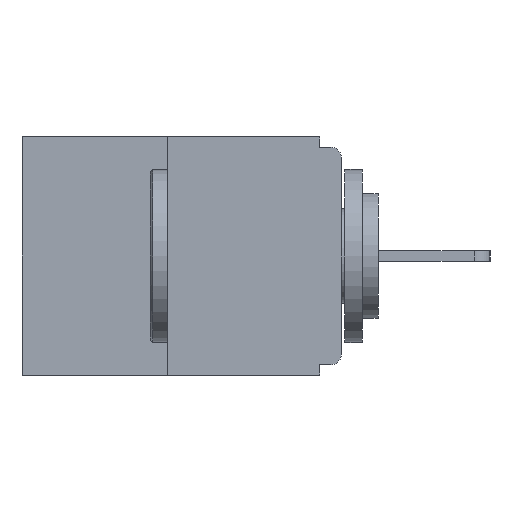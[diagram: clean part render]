
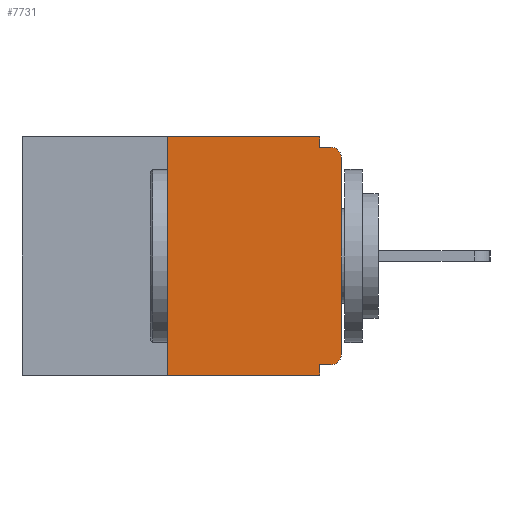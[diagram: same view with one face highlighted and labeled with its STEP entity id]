
A CAD part, left-side view. The second image highlights one B-rep face of the part: STEP entity #7731.
In plain terms, the highlighted planar face has unit normal (-1, 0, 0).
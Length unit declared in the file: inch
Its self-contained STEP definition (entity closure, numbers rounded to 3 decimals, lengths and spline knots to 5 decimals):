
#279 = VECTOR ( 'NONE', #20428, 39.37008 ) ;
#307 = CARTESIAN_POINT ( 'NONE',  ( 0., 0.015, -0.03 ) ) ;
#452 = DIRECTION ( 'NONE',  ( 0., -1., 0. ) ) ;
#669 = ORIENTED_EDGE ( 'NONE', *, *, #16260, .T. ) ;
#897 = VECTOR ( 'NONE', #19097, 39.37008 ) ;
#960 = EDGE_CURVE ( 'NONE', #13443, #11929, #16025, .T. ) ;
#2563 = DIRECTION ( 'NONE',  ( 0., 0., -1. ) ) ;
#2791 = CARTESIAN_POINT ( 'NONE',  ( 0., 0.46, 0. ) ) ;
#3746 = VERTEX_POINT ( 'NONE', #24439 ) ;
#3871 = VECTOR ( 'NONE', #7969, 39.37008 ) ;
#4039 = CARTESIAN_POINT ( 'NONE',  ( 0., 0., -0.328 ) ) ;
#4362 = EDGE_CURVE ( 'NONE', #23998, #17285, #21776, .T. ) ;
#4954 = VERTEX_POINT ( 'NONE', #19949 ) ;
#5020 = DIRECTION ( 'NONE',  ( 0., -1., 0. ) ) ;
#6920 = CARTESIAN_POINT ( 'NONE',  ( 0., 0.031, -0.015 ) ) ;
#7117 = CARTESIAN_POINT ( 'NONE',  ( 0., 0., -0.313 ) ) ;
#7198 = CARTESIAN_POINT ( 'NONE',  ( 0., 0., -0.015 ) ) ;
#7251 = EDGE_CURVE ( 'NONE', #3746, #13443, #26255, .T. ) ;
#7542 = CIRCLE ( 'NONE', #22063, 0.015 ) ;
#7731 = ADVANCED_FACE ( 'NONE', ( #13949 ), #19014, .F. ) ;
#7797 = CARTESIAN_POINT ( 'NONE',  ( 0., 0.031, -0.343 ) ) ;
#7969 = DIRECTION ( 'NONE',  ( 0., 0., -1. ) ) ;
#8011 = ORIENTED_EDGE ( 'NONE', *, *, #960, .T. ) ;
#8301 = ORIENTED_EDGE ( 'NONE', *, *, #15747, .F. ) ;
#8677 = VECTOR ( 'NONE', #17443, 39.37008 ) ;
#8935 = VERTEX_POINT ( 'NONE', #6920 ) ;
#9076 = DIRECTION ( 'NONE',  ( 0., 0., 1. ) ) ;
#10127 = VERTEX_POINT ( 'NONE', #22144 ) ;
#10469 = CARTESIAN_POINT ( 'NONE',  ( 0., 0., 0. ) ) ;
#10953 = CARTESIAN_POINT ( 'NONE',  ( 0., 0.46, -0.343 ) ) ;
#11827 = VECTOR ( 'NONE', #9076, 39.37008 ) ;
#11851 = LINE ( 'NONE', #4039, #897 ) ;
#11905 = LINE ( 'NONE', #18206, #279 ) ;
#11929 = VERTEX_POINT ( 'NONE', #25073 ) ;
#11999 = CARTESIAN_POINT ( 'NONE',  ( 0., 0.031, -0.328 ) ) ;
#12532 = VECTOR ( 'NONE', #19313, 39.37008 ) ;
#12934 = EDGE_CURVE ( 'NONE', #10127, #23942, #11905, .T. ) ;
#13120 = VERTEX_POINT ( 'NONE', #27563 ) ;
#13443 = VERTEX_POINT ( 'NONE', #7117 ) ;
#13949 = FACE_OUTER_BOUND ( 'NONE', #22352, .T. ) ;
#15265 = CARTESIAN_POINT ( 'NONE',  ( 0., 0.031, -0.343 ) ) ;
#15398 = DIRECTION ( 'NONE',  ( -1., 0., 0. ) ) ;
#15747 = EDGE_CURVE ( 'NONE', #23942, #13120, #18740, .T. ) ;
#16025 = LINE ( 'NONE', #10469, #11827 ) ;
#16260 = EDGE_CURVE ( 'NONE', #10127, #17285, #25893, .T. ) ;
#17071 = CARTESIAN_POINT ( 'NONE',  ( 0., 0.031, 0. ) ) ;
#17267 = ORIENTED_EDGE ( 'NONE', *, *, #12934, .F. ) ;
#17285 = VERTEX_POINT ( 'NONE', #15265 ) ;
#17443 = DIRECTION ( 'NONE',  ( 0., -1., 0. ) ) ;
#18043 = VECTOR ( 'NONE', #5020, 39.37008 ) ;
#18079 = DIRECTION ( 'NONE',  ( 0., 0., -1. ) ) ;
#18117 = DIRECTION ( 'NONE',  ( -1., 0., 0. ) ) ;
#18149 = DIRECTION ( 'NONE',  ( 0., 0., -1. ) ) ;
#18206 = CARTESIAN_POINT ( 'NONE',  ( 0., 0.25, 0. ) ) ;
#18212 = CARTESIAN_POINT ( 'NONE',  ( 0., 0.015, -0.313 ) ) ;
#18740 = LINE ( 'NONE', #2791, #18043 ) ;
#19014 = PLANE ( 'NONE',  #19746 ) ;
#19097 = DIRECTION ( 'NONE',  ( 0., 1., 0. ) ) ;
#19206 = DIRECTION ( 'NONE',  ( 1., 0., 0. ) ) ;
#19313 = DIRECTION ( 'NONE',  ( 0., 0., -1. ) ) ;
#19746 = AXIS2_PLACEMENT_3D ( 'NONE', #21814, #19206, #18149 ) ;
#19949 = CARTESIAN_POINT ( 'NONE',  ( 0., 0.015, -0.015 ) ) ;
#20428 = DIRECTION ( 'NONE',  ( 0., 0., 1. ) ) ;
#20435 = EDGE_CURVE ( 'NONE', #8935, #4954, #21671, .T. ) ;
#20749 = ORIENTED_EDGE ( 'NONE', *, *, #21510, .T. ) ;
#21510 = EDGE_CURVE ( 'NONE', #11929, #4954, #7542, .T. ) ;
#21671 = LINE ( 'NONE', #7198, #26805 ) ;
#21776 = LINE ( 'NONE', #7797, #3871 ) ;
#21814 = CARTESIAN_POINT ( 'NONE',  ( 0., 0.46, 0. ) ) ;
#22063 = AXIS2_PLACEMENT_3D ( 'NONE', #307, #15398, #2563 ) ;
#22144 = CARTESIAN_POINT ( 'NONE',  ( 0., 0.25, -0.343 ) ) ;
#22285 = AXIS2_PLACEMENT_3D ( 'NONE', #18212, #18117, #18079 ) ;
#22352 = EDGE_LOOP ( 'NONE', ( #8301, #17267, #669, #26537, #24157, #26897, #8011, #20749, #24184, #25549 ) ) ;
#22555 = CARTESIAN_POINT ( 'NONE',  ( 0., 0.25, 0. ) ) ;
#23942 = VERTEX_POINT ( 'NONE', #22555 ) ;
#23998 = VERTEX_POINT ( 'NONE', #11999 ) ;
#24054 = LINE ( 'NONE', #17071, #12532 ) ;
#24157 = ORIENTED_EDGE ( 'NONE', *, *, #27458, .F. ) ;
#24184 = ORIENTED_EDGE ( 'NONE', *, *, #20435, .F. ) ;
#24439 = CARTESIAN_POINT ( 'NONE',  ( 0., 0.015, -0.328 ) ) ;
#25073 = CARTESIAN_POINT ( 'NONE',  ( 0., 0., -0.03 ) ) ;
#25549 = ORIENTED_EDGE ( 'NONE', *, *, #26996, .F. ) ;
#25893 = LINE ( 'NONE', #10953, #8677 ) ;
#26255 = CIRCLE ( 'NONE', #22285, 0.015 ) ;
#26537 = ORIENTED_EDGE ( 'NONE', *, *, #4362, .F. ) ;
#26805 = VECTOR ( 'NONE', #452, 39.37008 ) ;
#26897 = ORIENTED_EDGE ( 'NONE', *, *, #7251, .T. ) ;
#26996 = EDGE_CURVE ( 'NONE', #13120, #8935, #24054, .T. ) ;
#27458 = EDGE_CURVE ( 'NONE', #3746, #23998, #11851, .T. ) ;
#27563 = CARTESIAN_POINT ( 'NONE',  ( 0., 0.031, 0. ) ) ;
